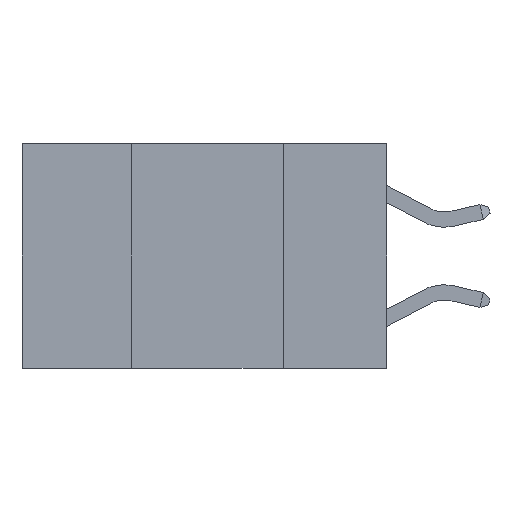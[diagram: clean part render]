
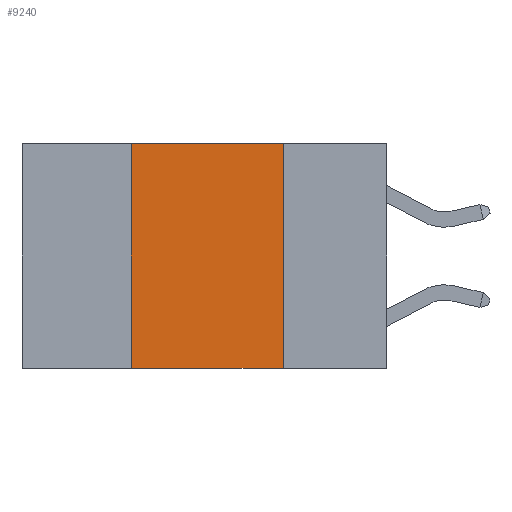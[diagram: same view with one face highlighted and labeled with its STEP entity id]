
A CAD part, left-side view. The second image highlights one B-rep face of the part: STEP entity #9240.
In plain terms, the highlighted planar face has unit normal (-1, 0, 0).
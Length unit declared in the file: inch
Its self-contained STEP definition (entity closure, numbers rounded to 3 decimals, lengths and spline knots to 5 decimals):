
#430 = DIRECTION ( 'NONE',  ( 0., -1., 0. ) ) ;
#505 = LINE ( 'NONE', #14916, #13985 ) ;
#670 = VERTEX_POINT ( 'NONE', #11808 ) ;
#740 = CARTESIAN_POINT ( 'NONE',  ( 0., 0.42, -0.37 ) ) ;
#998 = VERTEX_POINT ( 'NONE', #1861 ) ;
#1861 = CARTESIAN_POINT ( 'NONE',  ( 0., 0.42, 0. ) ) ;
#2394 = CARTESIAN_POINT ( 'NONE',  ( 0., 0.6, -0.37 ) ) ;
#4004 = ORIENTED_EDGE ( 'NONE', *, *, #14347, .F. ) ;
#4782 = CARTESIAN_POINT ( 'NONE',  ( 0., 0.6, 0. ) ) ;
#5126 = FACE_OUTER_BOUND ( 'NONE', #8209, .T. ) ;
#5628 = LINE ( 'NONE', #7353, #9796 ) ;
#6432 = VECTOR ( 'NONE', #13071, 39.37008 ) ;
#6511 = DIRECTION ( 'NONE',  ( 0., 0., -1. ) ) ;
#6839 = CARTESIAN_POINT ( 'NONE',  ( 0., 0.17, 0. ) ) ;
#6961 = LINE ( 'NONE', #18321, #6432 ) ;
#7353 = CARTESIAN_POINT ( 'NONE',  ( 0., 0.6, 0. ) ) ;
#8209 = EDGE_LOOP ( 'NONE', ( #15093, #8682, #4004, #16781 ) ) ;
#8682 = ORIENTED_EDGE ( 'NONE', *, *, #15419, .F. ) ;
#9240 = ADVANCED_FACE ( 'NONE', ( #5126 ), #15380, .F. ) ;
#9453 = DIRECTION ( 'NONE',  ( 0., -1., 0. ) ) ;
#9602 = EDGE_CURVE ( 'NONE', #19585, #670, #18591, .T. ) ;
#9796 = VECTOR ( 'NONE', #430, 39.37008 ) ;
#11808 = CARTESIAN_POINT ( 'NONE',  ( 0., 0.17, -0.37 ) ) ;
#13071 = DIRECTION ( 'NONE',  ( 0., 0., -1. ) ) ;
#13985 = VECTOR ( 'NONE', #21810, 39.37008 ) ;
#14347 = EDGE_CURVE ( 'NONE', #19585, #998, #505, .T. ) ;
#14916 = CARTESIAN_POINT ( 'NONE',  ( 0., 0.42, 0. ) ) ;
#15093 = ORIENTED_EDGE ( 'NONE', *, *, #15556, .F. ) ;
#15380 = PLANE ( 'NONE',  #16295 ) ;
#15419 = EDGE_CURVE ( 'NONE', #998, #20683, #5628, .T. ) ;
#15556 = EDGE_CURVE ( 'NONE', #20683, #670, #6961, .T. ) ;
#16295 = AXIS2_PLACEMENT_3D ( 'NONE', #4782, #17128, #6511 ) ;
#16781 = ORIENTED_EDGE ( 'NONE', *, *, #9602, .T. ) ;
#17128 = DIRECTION ( 'NONE',  ( 1., 0., 0. ) ) ;
#18048 = VECTOR ( 'NONE', #9453, 39.37008 ) ;
#18321 = CARTESIAN_POINT ( 'NONE',  ( 0., 0.17, 0. ) ) ;
#18591 = LINE ( 'NONE', #2394, #18048 ) ;
#19585 = VERTEX_POINT ( 'NONE', #740 ) ;
#20683 = VERTEX_POINT ( 'NONE', #6839 ) ;
#21810 = DIRECTION ( 'NONE',  ( 0., 0., 1. ) ) ;
